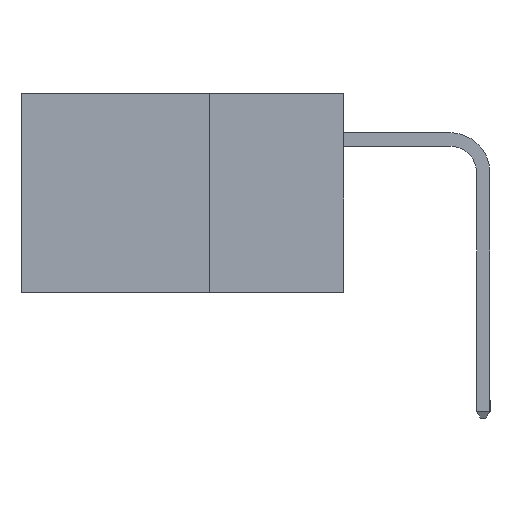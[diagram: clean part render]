
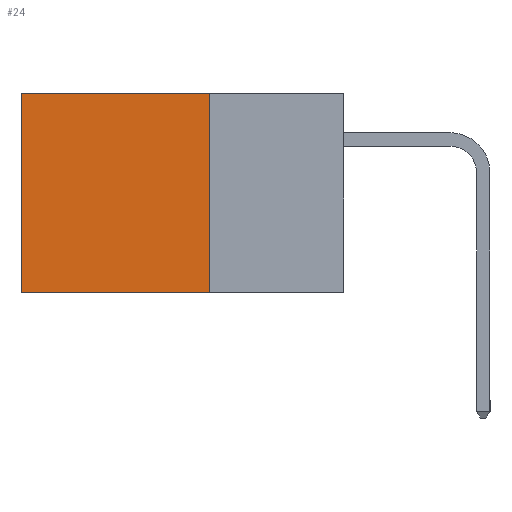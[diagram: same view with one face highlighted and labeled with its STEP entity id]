
A CAD part, left-side view. The second image highlights one B-rep face of the part: STEP entity #24.
In plain terms, the highlighted planar face has unit normal (-1, 0, 0).
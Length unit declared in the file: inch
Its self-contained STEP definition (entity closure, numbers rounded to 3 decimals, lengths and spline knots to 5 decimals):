
#20 = CARTESIAN_POINT ( 'NONE',  ( 0.2615, 0.25, -0.37 ) ) ;
#24 = ADVANCED_FACE ( 'NONE', ( #206 ), #3886, .F. ) ;
#206 = FACE_OUTER_BOUND ( 'NONE', #510, .T. ) ;
#510 = EDGE_LOOP ( 'NONE', ( #9350, #1790, #3830, #7769 ) ) ;
#579 = LINE ( 'NONE', #5565, #4689 ) ;
#825 = VERTEX_POINT ( 'NONE', #3283 ) ;
#1035 = DIRECTION ( 'NONE',  ( 0., 0., -1. ) ) ;
#1327 = VERTEX_POINT ( 'NONE', #9730 ) ;
#1790 = ORIENTED_EDGE ( 'NONE', *, *, #9033, .F. ) ;
#2157 = VECTOR ( 'NONE', #8781, 39.37008 ) ;
#2259 = VERTEX_POINT ( 'NONE', #5683 ) ;
#2863 = CARTESIAN_POINT ( 'NONE',  ( 0.2615, 0.25, -0.37 ) ) ;
#3283 = CARTESIAN_POINT ( 'NONE',  ( 0.2615, 0.25, -0.37 ) ) ;
#3470 = VERTEX_POINT ( 'NONE', #6872 ) ;
#3817 = AXIS2_PLACEMENT_3D ( 'NONE', #8772, #7531, #1035 ) ;
#3830 = ORIENTED_EDGE ( 'NONE', *, *, #6797, .F. ) ;
#3886 = PLANE ( 'NONE',  #3817 ) ;
#3899 = VECTOR ( 'NONE', #8739, 39.37008 ) ;
#4212 = LINE ( 'NONE', #8758, #2157 ) ;
#4662 = LINE ( 'NONE', #20, #8300 ) ;
#4689 = VECTOR ( 'NONE', #5548, 39.37008 ) ;
#4841 = EDGE_CURVE ( 'NONE', #2259, #1327, #4212, .T. ) ;
#5258 = EDGE_CURVE ( 'NONE', #1327, #3470, #579, .T. ) ;
#5548 = DIRECTION ( 'NONE',  ( 0., 0., -1. ) ) ;
#5565 = CARTESIAN_POINT ( 'NONE',  ( 0.2615, 0.6, -0.37 ) ) ;
#5683 = CARTESIAN_POINT ( 'NONE',  ( 0.2615, 0.25, 0. ) ) ;
#6139 = LINE ( 'NONE', #2863, #3899 ) ;
#6797 = EDGE_CURVE ( 'NONE', #2259, #825, #4662, .T. ) ;
#6872 = CARTESIAN_POINT ( 'NONE',  ( 0.2615, 0.6, -0.37 ) ) ;
#7531 = DIRECTION ( 'NONE',  ( 1., 0., 0. ) ) ;
#7769 = ORIENTED_EDGE ( 'NONE', *, *, #4841, .T. ) ;
#8245 = DIRECTION ( 'NONE',  ( 0., 0., -1. ) ) ;
#8300 = VECTOR ( 'NONE', #8245, 39.37008 ) ;
#8739 = DIRECTION ( 'NONE',  ( 0., 1., 0. ) ) ;
#8758 = CARTESIAN_POINT ( 'NONE',  ( 0.2615, 0.25, 0. ) ) ;
#8772 = CARTESIAN_POINT ( 'NONE',  ( 0.2615, 0.25, -0.37 ) ) ;
#8781 = DIRECTION ( 'NONE',  ( 0., 1., 0. ) ) ;
#9033 = EDGE_CURVE ( 'NONE', #825, #3470, #6139, .T. ) ;
#9350 = ORIENTED_EDGE ( 'NONE', *, *, #5258, .T. ) ;
#9730 = CARTESIAN_POINT ( 'NONE',  ( 0.2615, 0.6, 0. ) ) ;
